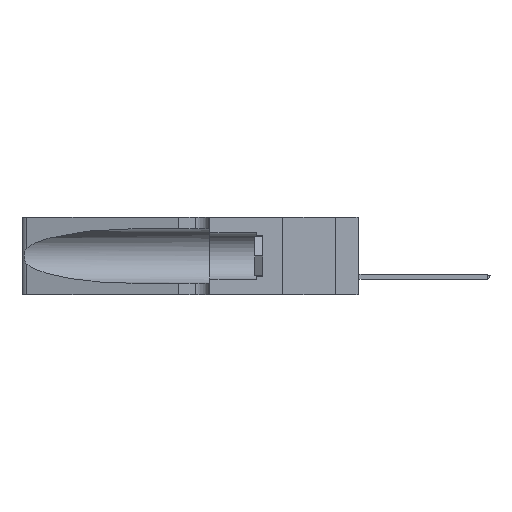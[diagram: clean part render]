
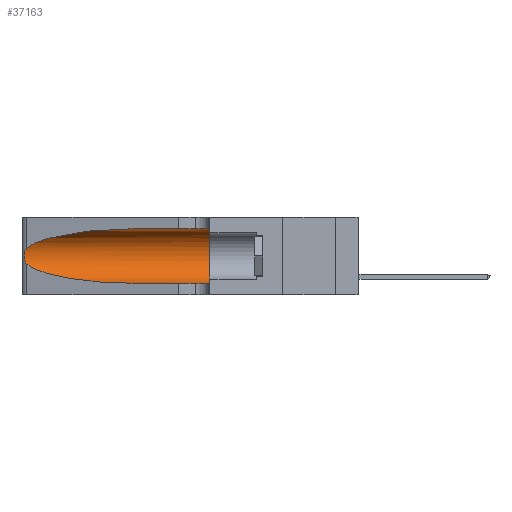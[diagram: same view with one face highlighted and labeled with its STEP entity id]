
A CAD part, left-side view. The second image highlights one B-rep face of the part: STEP entity #37163.
In plain terms, the highlighted cylindrical face has radius 3.308 mm (diameter 6.617 mm), a partial arc.
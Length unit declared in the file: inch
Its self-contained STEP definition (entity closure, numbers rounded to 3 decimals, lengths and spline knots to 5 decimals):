
#761 = CARTESIAN_POINT ( 'NONE',  ( 0.2373, 1.15595, 0.28018 ) ) ;
#1028 = CARTESIAN_POINT ( 'NONE',  ( 0.1305, 0.35, 0.185 ) ) ;
#3938 = CARTESIAN_POINT ( 'NONE',  ( 0.25787, 1.23484, 0.2124 ) ) ;
#6680 =( BOUNDED_CURVE ( )  B_SPLINE_CURVE ( 3, ( #9086, #33391, #16429, #16593 ),
 .UNSPECIFIED., .F., .T. ) 
 B_SPLINE_CURVE_WITH_KNOTS ( ( 4, 4 ),
 ( 3.44316, 4.71239 ),
 .UNSPECIFIED. ) 
 CURVE ( )  GEOMETRIC_REPRESENTATION_ITEM ( )  RATIONAL_B_SPLINE_CURVE ( ( 1., 0.87, 0.87, 1. ) ) 
 REPRESENTATION_ITEM ( '' )  );
#8133 = CARTESIAN_POINT ( 'NONE',  ( 0.25555, 1.22994, 0.2215 ) ) ;
#8483 = EDGE_LOOP ( 'NONE', ( #44653, #50313, #25306, #15923, #14944, #20309 ) ) ;
#9086 = CARTESIAN_POINT ( 'NONE',  ( 0.25487, 1.22718, 0.14631 ) ) ;
#10052 = DIRECTION ( 'NONE',  ( 0., -1., 0. ) ) ;
#11671 = CARTESIAN_POINT ( 'NONE',  ( 0.25487, 1.22718, 0.22369 ) ) ;
#11991 = CARTESIAN_POINT ( 'NONE',  ( 0.26018, 1.23835, 0.19895 ) ) ;
#13297 = CARTESIAN_POINT ( 'NONE',  ( 0.25487, 1.22718, 0.22369 ) ) ;
#13412 =( BOUNDED_CURVE ( )  B_SPLINE_CURVE ( 3, ( #41541, #37649, #761, #13297 ),
 .UNSPECIFIED., .F., .F. ) 
 B_SPLINE_CURVE_WITH_KNOTS ( ( 4, 4 ),
 ( 1.5708, 2.84003 ),
 .UNSPECIFIED. ) 
 CURVE ( )  GEOMETRIC_REPRESENTATION_ITEM ( )  RATIONAL_B_SPLINE_CURVE ( ( 1., 0.87, 0.87, 1. ) ) 
 REPRESENTATION_ITEM ( '' )  );
#14944 = ORIENTED_EDGE ( 'NONE', *, *, #30435, .F. ) ;
#15776 = CARTESIAN_POINT ( 'NONE',  ( 0.26017, 1.23833, 0.17102 ) ) ;
#15923 = ORIENTED_EDGE ( 'NONE', *, *, #16522, .T. ) ;
#16103 = CARTESIAN_POINT ( 'NONE',  ( 0.25856, 1.23593, 0.16098 ) ) ;
#16429 = CARTESIAN_POINT ( 'NONE',  ( 0.18966, 0.96281, 0.05475 ) ) ;
#16522 = EDGE_CURVE ( 'NONE', #21359, #17061, #32548, .T. ) ;
#16593 = CARTESIAN_POINT ( 'NONE',  ( 0.1305, 0.72297, 0.05475 ) ) ;
#16669 = CYLINDRICAL_SURFACE ( 'NONE', #28018, 0.13025 ) ;
#17061 = VERTEX_POINT ( 'NONE', #18280 ) ;
#17183 = CIRCLE ( 'NONE', #18276, 0.13025 ) ;
#18276 = AXIS2_PLACEMENT_3D ( 'NONE', #1028, #41637, #45697 ) ;
#18280 = CARTESIAN_POINT ( 'NONE',  ( 0.1305, 0.35, 0.05475 ) ) ;
#19295 = FACE_OUTER_BOUND ( 'NONE', #8483, .T. ) ;
#19692 = CARTESIAN_POINT ( 'NONE',  ( 0.25789, 1.23486, 0.15765 ) ) ;
#20309 = ORIENTED_EDGE ( 'NONE', *, *, #42934, .F. ) ;
#21359 = VERTEX_POINT ( 'NONE', #32711 ) ;
#21379 = LINE ( 'NONE', #22565, #44292 ) ;
#21522 = VERTEX_POINT ( 'NONE', #51057 ) ;
#21830 = DIRECTION ( 'NONE',  ( 0., -1., 0. ) ) ;
#22565 = CARTESIAN_POINT ( 'NONE',  ( 0.1305, 1.61858, 0.31525 ) ) ;
#22899 = CARTESIAN_POINT ( 'NONE',  ( 0.1305, 1.61858, 0.05475 ) ) ;
#24265 = CARTESIAN_POINT ( 'NONE',  ( 0.25854, 1.2359, 0.20912 ) ) ;
#25306 = ORIENTED_EDGE ( 'NONE', *, *, #48751, .T. ) ;
#28018 = AXIS2_PLACEMENT_3D ( 'NONE', #50651, #10052, #30479 ) ;
#30435 = EDGE_CURVE ( 'NONE', #33653, #17061, #17183, .T. ) ;
#30479 = DIRECTION ( 'NONE',  ( 0., 0., -1. ) ) ;
#30501 = VERTEX_POINT ( 'NONE', #38469 ) ;
#31786 = EDGE_CURVE ( 'NONE', #21522, #47488, #13412, .T. ) ;
#32548 = LINE ( 'NONE', #22899, #44042 ) ;
#32637 = CARTESIAN_POINT ( 'NONE',  ( 0.1305, 0.35, 0.31525 ) ) ;
#32711 = CARTESIAN_POINT ( 'NONE',  ( 0.1305, 0.72297, 0.05475 ) ) ;
#33391 = CARTESIAN_POINT ( 'NONE',  ( 0.2373, 1.15595, 0.08982 ) ) ;
#33653 = VERTEX_POINT ( 'NONE', #32637 ) ;
#36505 = CARTESIAN_POINT ( 'NONE',  ( 0.25487, 1.22718, 0.14631 ) ) ;
#36679 = CARTESIAN_POINT ( 'NONE',  ( 0.26075, 1.23896, 0.19203 ) ) ;
#37163 = ADVANCED_FACE ( 'NONE', ( #19295 ), #16669, .F. ) ;
#37649 = CARTESIAN_POINT ( 'NONE',  ( 0.18966, 0.96281, 0.31525 ) ) ;
#37855 = B_SPLINE_CURVE_WITH_KNOTS ( 'NONE', 3,
 ( #11671, #8133, #48358, #3938, #24265, #11991, #36679, #40441, #15776, #16103, #19692, #48018, #44479, #36505 ),
 .UNSPECIFIED., .F., .F.,
 ( 4, 2, 2, 2, 2, 2, 4 ),
 ( 0., 0.00027, 0.00053, 0.00107, 0.0016, 0.00187, 0.00214 ),
 .UNSPECIFIED. ) ;
#38469 = CARTESIAN_POINT ( 'NONE',  ( 0.25487, 1.22718, 0.14631 ) ) ;
#39819 = CARTESIAN_POINT ( 'NONE',  ( 0.25487, 1.22718, 0.22369 ) ) ;
#40441 = CARTESIAN_POINT ( 'NONE',  ( 0.26075, 1.23896, 0.178 ) ) ;
#41541 = CARTESIAN_POINT ( 'NONE',  ( 0.1305, 0.72297, 0.31525 ) ) ;
#41637 = DIRECTION ( 'NONE',  ( 0., 1., 0. ) ) ;
#42934 = EDGE_CURVE ( 'NONE', #21522, #33653, #21379, .T. ) ;
#44042 = VECTOR ( 'NONE', #51262, 39.37008 ) ;
#44292 = VECTOR ( 'NONE', #21830, 39.37008 ) ;
#44479 = CARTESIAN_POINT ( 'NONE',  ( 0.25555, 1.22993, 0.14849 ) ) ;
#44653 = ORIENTED_EDGE ( 'NONE', *, *, #31786, .T. ) ;
#45697 = DIRECTION ( 'NONE',  ( 0., 0., 1. ) ) ;
#47488 = VERTEX_POINT ( 'NONE', #39819 ) ;
#48018 = CARTESIAN_POINT ( 'NONE',  ( 0.25639, 1.23186, 0.15144 ) ) ;
#48358 = CARTESIAN_POINT ( 'NONE',  ( 0.25639, 1.23184, 0.21858 ) ) ;
#48751 = EDGE_CURVE ( 'NONE', #30501, #21359, #6680, .T. ) ;
#50313 = ORIENTED_EDGE ( 'NONE', *, *, #51669, .T. ) ;
#50651 = CARTESIAN_POINT ( 'NONE',  ( 0.1305, 1.61858, 0.185 ) ) ;
#51057 = CARTESIAN_POINT ( 'NONE',  ( 0.1305, 0.72297, 0.31525 ) ) ;
#51262 = DIRECTION ( 'NONE',  ( 0., -1., 0. ) ) ;
#51669 = EDGE_CURVE ( 'NONE', #47488, #30501, #37855, .T. ) ;
